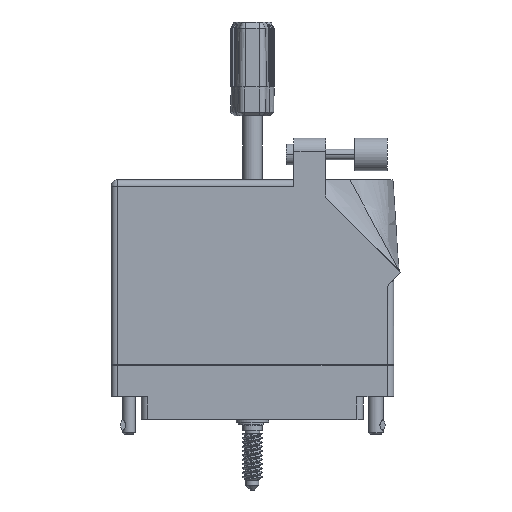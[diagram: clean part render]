
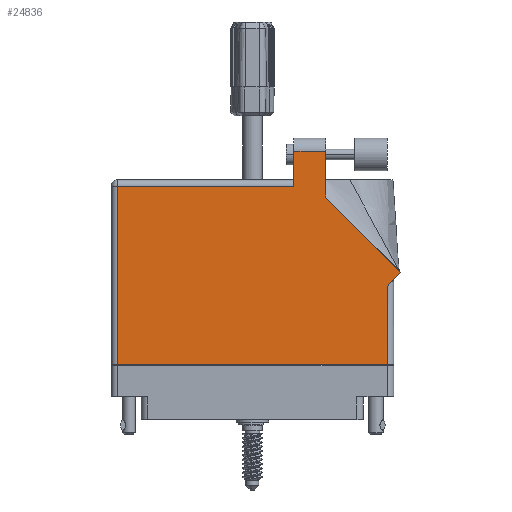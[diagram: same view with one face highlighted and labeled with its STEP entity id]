
A CAD part, front view. The second image highlights one B-rep face of the part: STEP entity #24836.
In plain terms, the highlighted face is planar.
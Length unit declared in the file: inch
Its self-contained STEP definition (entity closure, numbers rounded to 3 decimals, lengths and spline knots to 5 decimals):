
#1483 = DIRECTION ( 'NONE',  ( 1., 0., 0. ) ) ;
#2990 = VERTEX_POINT ( 'NONE', #84872 ) ;
#3358 = LINE ( 'NONE', #45019, #7824 ) ;
#3814 = PLANE ( 'NONE',  #30055 ) ;
#4550 = VECTOR ( 'NONE', #68219, 39.37008 ) ;
#4956 = ORIENTED_EDGE ( 'NONE', *, *, #91042, .T. ) ;
#6356 = EDGE_LOOP ( 'NONE', ( #33777, #84851, #67110, #77274, #89996, #9220, #4956, #15718, #44673 ) ) ;
#7482 = CARTESIAN_POINT ( 'NONE',  ( 1.297, 0.715, 0.617 ) ) ;
#7824 = VECTOR ( 'NONE', #45615, 39.37008 ) ;
#8241 = DIRECTION ( 'NONE',  ( -1., 0., 0. ) ) ;
#9220 = ORIENTED_EDGE ( 'NONE', *, *, #25159, .T. ) ;
#9368 = EDGE_CURVE ( 'NONE', #86804, #2990, #67797, .T. ) ;
#10307 = VERTEX_POINT ( 'NONE', #36871 ) ;
#10833 = CARTESIAN_POINT ( 'NONE',  ( 0.399, 1.675, 0.617 ) ) ;
#11166 = CARTESIAN_POINT ( 'NONE',  ( 1.42971, 0.78571, 0.617 ) ) ;
#14326 = LINE ( 'NONE', #7482, #27510 ) ;
#15718 = ORIENTED_EDGE ( 'NONE', *, *, #23448, .T. ) ;
#19118 = EDGE_CURVE ( 'NONE', #10307, #69921, #52606, .T. ) ;
#20214 = EDGE_CURVE ( 'NONE', #69749, #43910, #29293, .T. ) ;
#21615 = VECTOR ( 'NONE', #22585, 39.37008 ) ;
#22585 = DIRECTION ( 'NONE',  ( 0., -1., 0. ) ) ;
#23141 = EDGE_CURVE ( 'NONE', #51409, #69749, #29924, .T. ) ;
#23448 = EDGE_CURVE ( 'NONE', #54660, #86804, #3358, .T. ) ;
#23669 = VECTOR ( 'NONE', #24883, 39.37008 ) ;
#24836 = ADVANCED_FACE ( 'NONE', ( #64857 ), #3814, .F. ) ;
#24883 = DIRECTION ( 'NONE',  ( 0., 1., 0. ) ) ;
#25159 = EDGE_CURVE ( 'NONE', #43910, #51461, #78056, .T. ) ;
#27510 = VECTOR ( 'NONE', #57674, 39.37008 ) ;
#29293 = LINE ( 'NONE', #57096, #21615 ) ;
#29924 = LINE ( 'NONE', #74704, #4550 ) ;
#30055 = AXIS2_PLACEMENT_3D ( 'NONE', #38940, #45128, #59245 ) ;
#31180 = DIRECTION ( 'NONE',  ( 0., -1., 0. ) ) ;
#31910 = DIRECTION ( 'NONE',  ( -0.707, 0.707, 0. ) ) ;
#32844 = CARTESIAN_POINT ( 'NONE',  ( 0.399, 1.613, 0.617 ) ) ;
#33777 = ORIENTED_EDGE ( 'NONE', *, *, #64603, .T. ) ;
#36871 = CARTESIAN_POINT ( 'NONE',  ( 0.706, 1.95, 0.617 ) ) ;
#38316 = VECTOR ( 'NONE', #1483, 39.37008 ) ;
#38940 = CARTESIAN_POINT ( 'NONE',  ( -1.359, 1.675, 0.617 ) ) ;
#43583 = LINE ( 'NONE', #60328, #23669 ) ;
#43910 = VERTEX_POINT ( 'NONE', #75049 ) ;
#44673 = ORIENTED_EDGE ( 'NONE', *, *, #9368, .T. ) ;
#45019 = CARTESIAN_POINT ( 'NONE',  ( 1.359, 0.715, 0.617 ) ) ;
#45128 = DIRECTION ( 'NONE',  ( 0., 0., -1. ) ) ;
#45615 = DIRECTION ( 'NONE',  ( 0.707, 0.707, 0. ) ) ;
#48220 = VECTOR ( 'NONE', #8241, 39.37008 ) ;
#50100 = CARTESIAN_POINT ( 'NONE',  ( 1.42971, 0.78571, 0.617 ) ) ;
#51409 = VERTEX_POINT ( 'NONE', #32844 ) ;
#51461 = VERTEX_POINT ( 'NONE', #76590 ) ;
#52606 = LINE ( 'NONE', #71403, #48220 ) ;
#54121 = VECTOR ( 'NONE', #31180, 39.37008 ) ;
#54660 = VERTEX_POINT ( 'NONE', #63793 ) ;
#57096 = CARTESIAN_POINT ( 'NONE',  ( -1.297, -0.1, 0.617 ) ) ;
#57674 = DIRECTION ( 'NONE',  ( 0., 1., 0. ) ) ;
#59245 = DIRECTION ( 'NONE',  ( -1., 0., 0. ) ) ;
#59731 = CARTESIAN_POINT ( 'NONE',  ( -1.297, 1.613, 0.617 ) ) ;
#60328 = CARTESIAN_POINT ( 'NONE',  ( 0.706, 1.50942, 0.617 ) ) ;
#62029 = CARTESIAN_POINT ( 'NONE',  ( -1.359, -0.1, 0.617 ) ) ;
#63793 = CARTESIAN_POINT ( 'NONE',  ( 1.297, 0.653, 0.617 ) ) ;
#64473 = VECTOR ( 'NONE', #31910, 39.37008 ) ;
#64603 = EDGE_CURVE ( 'NONE', #2990, #10307, #43583, .T. ) ;
#64857 = FACE_OUTER_BOUND ( 'NONE', #6356, .T. ) ;
#67110 = ORIENTED_EDGE ( 'NONE', *, *, #71003, .T. ) ;
#67797 = LINE ( 'NONE', #50100, #64473 ) ;
#68219 = DIRECTION ( 'NONE',  ( -1., 0., 0. ) ) ;
#69749 = VERTEX_POINT ( 'NONE', #59731 ) ;
#69921 = VERTEX_POINT ( 'NONE', #74562 ) ;
#71003 = EDGE_CURVE ( 'NONE', #69921, #51409, #72857, .T. ) ;
#71403 = CARTESIAN_POINT ( 'NONE',  ( 0.399, 1.95, 0.617 ) ) ;
#72857 = LINE ( 'NONE', #10833, #54121 ) ;
#74562 = CARTESIAN_POINT ( 'NONE',  ( 0.399, 1.95, 0.617 ) ) ;
#74704 = CARTESIAN_POINT ( 'NONE',  ( -1.359, 1.613, 0.617 ) ) ;
#75049 = CARTESIAN_POINT ( 'NONE',  ( -1.297, -0.1, 0.617 ) ) ;
#76590 = CARTESIAN_POINT ( 'NONE',  ( 1.297, -0.1, 0.617 ) ) ;
#77274 = ORIENTED_EDGE ( 'NONE', *, *, #23141, .T. ) ;
#78056 = LINE ( 'NONE', #62029, #38316 ) ;
#84851 = ORIENTED_EDGE ( 'NONE', *, *, #19118, .T. ) ;
#84872 = CARTESIAN_POINT ( 'NONE',  ( 0.706, 1.50942, 0.617 ) ) ;
#86804 = VERTEX_POINT ( 'NONE', #11166 ) ;
#89996 = ORIENTED_EDGE ( 'NONE', *, *, #20214, .T. ) ;
#91042 = EDGE_CURVE ( 'NONE', #51461, #54660, #14326, .T. ) ;
